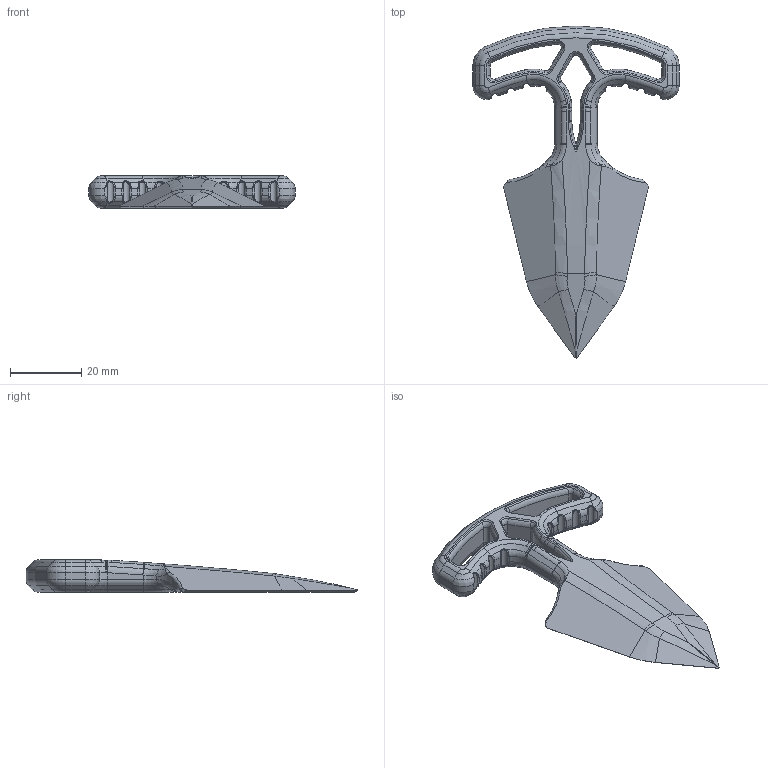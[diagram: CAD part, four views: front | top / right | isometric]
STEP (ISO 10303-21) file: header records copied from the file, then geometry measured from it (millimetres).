
FILE_DESCRIPTION(/* description */ (''),/* implementation_level */ '2;1');
FILE_NAME(/* name */ 'Survive.step',/* time_stamp */ '2021-10-14T20:38:45-04:00',/* author */ (''),/* organization */ (''),/* preprocessor_version */ 'ST-DEVELOPER v18.1',/* originating_system */ 'Autodesk Translation Framework v10.10.0.1391',/* authorisation */ '');
FILE_SCHEMA (('AUTOMOTIVE_DESIGN { 1 0 10303 214 3 1 1 }'));
Length unit declared in the file: millimetre
Products named in the file (1): Survive
Bounding box: 58 x 93.32 x 9 mm (x, y, z)
Volume: 11908.2 mm3; surface area: 7683.3 mm2
Topology: 1 solids, 5 shells, 522 faces, 1249 edges, 699 vertices
Faces by surface type: bspline 189, cylinder 116, torus 90, cone 70, plane 57
Full cylindrical faces by diameter (mm): 17.5 x1, 22 x1
Entity records: 18762 total; most frequent: CARTESIAN_POINT 7861, ORIENTED_EDGE 2424, DIRECTION 2038, EDGE_CURVE 1212, AXIS2_PLACEMENT_3D 868, VERTEX_POINT 699, EDGE_LOOP 529, FACE_OUTER_BOUND 522
